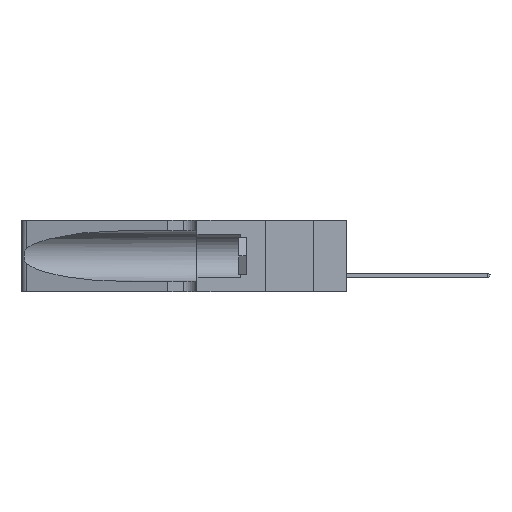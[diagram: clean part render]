
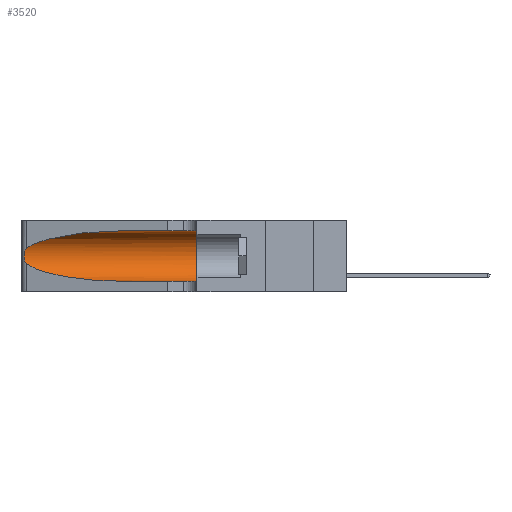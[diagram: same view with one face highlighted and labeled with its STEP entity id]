
A CAD part, left-side view. The second image highlights one B-rep face of the part: STEP entity #3520.
In plain terms, the highlighted cylindrical face has radius 3.308 mm (diameter 6.617 mm), a partial arc.
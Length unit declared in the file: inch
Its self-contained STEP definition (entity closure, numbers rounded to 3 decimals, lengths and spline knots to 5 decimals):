
#1212 = VECTOR ( 'NONE', #15139, 39.37008 ) ;
#1886 =( BOUNDED_CURVE ( )  B_SPLINE_CURVE ( 3, ( #22516, #39188, #35856, #42507 ),
 .UNSPECIFIED., .F., .T. ) 
 B_SPLINE_CURVE_WITH_KNOTS ( ( 4, 4 ),
 ( 1.5708, 2.84003 ),
 .UNSPECIFIED. ) 
 CURVE ( )  GEOMETRIC_REPRESENTATION_ITEM ( )  RATIONAL_B_SPLINE_CURVE ( ( 1., 0.87, 0.87, 1. ) ) 
 REPRESENTATION_ITEM ( '' )  );
#2965 = FACE_OUTER_BOUND ( 'NONE', #38478, .T. ) ;
#3320 = ORIENTED_EDGE ( 'NONE', *, *, #29223, .T. ) ;
#3520 = ADVANCED_FACE ( 'NONE', ( #2965 ), #28859, .F. ) ;
#4287 = CARTESIAN_POINT ( 'NONE',  ( 0.18966, 0.96281, 0.05475 ) ) ;
#4423 = CARTESIAN_POINT ( 'NONE',  ( 0.1305, 0.35, 0.05475 ) ) ;
#4901 = CARTESIAN_POINT ( 'NONE',  ( 0.26017, 1.23833, 0.17102 ) ) ;
#5806 = VERTEX_POINT ( 'NONE', #4423 ) ;
#6596 = DIRECTION ( 'NONE',  ( 0., 1., 0. ) ) ;
#6726 = CARTESIAN_POINT ( 'NONE',  ( 0.1305, 0.35, 0.185 ) ) ;
#7223 = CARTESIAN_POINT ( 'NONE',  ( 0.1305, 1.61858, 0.31525 ) ) ;
#7584 = EDGE_CURVE ( 'NONE', #34844, #7941, #1886, .T. ) ;
#7763 =( BOUNDED_CURVE ( )  B_SPLINE_CURVE ( 3, ( #33825, #10805, #4287, #20912 ),
 .UNSPECIFIED., .F., .F. ) 
 B_SPLINE_CURVE_WITH_KNOTS ( ( 4, 4 ),
 ( 3.44316, 4.71239 ),
 .UNSPECIFIED. ) 
 CURVE ( )  GEOMETRIC_REPRESENTATION_ITEM ( )  RATIONAL_B_SPLINE_CURVE ( ( 1., 0.87, 0.87, 1. ) ) 
 REPRESENTATION_ITEM ( '' )  );
#7941 = VERTEX_POINT ( 'NONE', #16054 ) ;
#8264 = CARTESIAN_POINT ( 'NONE',  ( 0.25639, 1.23186, 0.15144 ) ) ;
#8314 = CARTESIAN_POINT ( 'NONE',  ( 0.1305, 0.35, 0.31525 ) ) ;
#9198 = VERTEX_POINT ( 'NONE', #40824 ) ;
#10805 = CARTESIAN_POINT ( 'NONE',  ( 0.2373, 1.15595, 0.08982 ) ) ;
#10886 = VECTOR ( 'NONE', #20127, 39.37008 ) ;
#11933 = AXIS2_PLACEMENT_3D ( 'NONE', #38541, #35711, #20340 ) ;
#12037 = CARTESIAN_POINT ( 'NONE',  ( 0.26075, 1.23896, 0.19203 ) ) ;
#15139 = DIRECTION ( 'NONE',  ( 0., -1., 0. ) ) ;
#15474 = CARTESIAN_POINT ( 'NONE',  ( 0.25639, 1.23184, 0.21858 ) ) ;
#15624 = ORIENTED_EDGE ( 'NONE', *, *, #26979, .T. ) ;
#15671 = VERTEX_POINT ( 'NONE', #30046 ) ;
#16045 = ORIENTED_EDGE ( 'NONE', *, *, #30670, .T. ) ;
#16054 = CARTESIAN_POINT ( 'NONE',  ( 0.25487, 1.22718, 0.22369 ) ) ;
#16184 = ORIENTED_EDGE ( 'NONE', *, *, #7584, .T. ) ;
#16254 = EDGE_CURVE ( 'NONE', #34844, #33401, #18668, .T. ) ;
#17661 = CARTESIAN_POINT ( 'NONE',  ( 0.1305, 0.72297, 0.31525 ) ) ;
#18661 = CARTESIAN_POINT ( 'NONE',  ( 0.25555, 1.22993, 0.14849 ) ) ;
#18668 = LINE ( 'NONE', #7223, #10886 ) ;
#18811 = EDGE_CURVE ( 'NONE', #33401, #5806, #36048, .T. ) ;
#18915 = LINE ( 'NONE', #35158, #1212 ) ;
#20127 = DIRECTION ( 'NONE',  ( 0., -1., 0. ) ) ;
#20340 = DIRECTION ( 'NONE',  ( 0., 0., -1. ) ) ;
#20912 = CARTESIAN_POINT ( 'NONE',  ( 0.1305, 0.72297, 0.05475 ) ) ;
#21403 = CARTESIAN_POINT ( 'NONE',  ( 0.25789, 1.23486, 0.15765 ) ) ;
#21866 = CARTESIAN_POINT ( 'NONE',  ( 0.25854, 1.2359, 0.20912 ) ) ;
#22516 = CARTESIAN_POINT ( 'NONE',  ( 0.1305, 0.72297, 0.31525 ) ) ;
#25321 = CARTESIAN_POINT ( 'NONE',  ( 0.26018, 1.23835, 0.19895 ) ) ;
#25450 = AXIS2_PLACEMENT_3D ( 'NONE', #6726, #6596, #32948 ) ;
#26979 = EDGE_CURVE ( 'NONE', #15671, #9198, #7763, .T. ) ;
#28859 = CYLINDRICAL_SURFACE ( 'NONE', #11933, 0.13025 ) ;
#29223 = EDGE_CURVE ( 'NONE', #7941, #15671, #29593, .T. ) ;
#29593 = B_SPLINE_CURVE_WITH_KNOTS ( 'NONE', 3,
 ( #31578, #35346, #15474, #41717, #21866, #25321, #12037, #41264, #4901, #41417, #21403, #8264, #18661, #41856 ),
 .UNSPECIFIED., .F., .F.,
 ( 4, 2, 2, 2, 2, 2, 4 ),
 ( 0., 0.00027, 0.00053, 0.00107, 0.0016, 0.00187, 0.00214 ),
 .UNSPECIFIED. ) ;
#30046 = CARTESIAN_POINT ( 'NONE',  ( 0.25487, 1.22718, 0.14631 ) ) ;
#30174 = ORIENTED_EDGE ( 'NONE', *, *, #18811, .F. ) ;
#30670 = EDGE_CURVE ( 'NONE', #9198, #5806, #18915, .T. ) ;
#31578 = CARTESIAN_POINT ( 'NONE',  ( 0.25487, 1.22718, 0.22369 ) ) ;
#32948 = DIRECTION ( 'NONE',  ( 0., 0., 1. ) ) ;
#33401 = VERTEX_POINT ( 'NONE', #8314 ) ;
#33825 = CARTESIAN_POINT ( 'NONE',  ( 0.25487, 1.22718, 0.14631 ) ) ;
#34844 = VERTEX_POINT ( 'NONE', #17661 ) ;
#35158 = CARTESIAN_POINT ( 'NONE',  ( 0.1305, 1.61858, 0.05475 ) ) ;
#35346 = CARTESIAN_POINT ( 'NONE',  ( 0.25555, 1.22994, 0.2215 ) ) ;
#35711 = DIRECTION ( 'NONE',  ( 0., -1., 0. ) ) ;
#35856 = CARTESIAN_POINT ( 'NONE',  ( 0.2373, 1.15595, 0.28018 ) ) ;
#36048 = CIRCLE ( 'NONE', #25450, 0.13025 ) ;
#38478 = EDGE_LOOP ( 'NONE', ( #16184, #3320, #15624, #16045, #30174, #42156 ) ) ;
#38541 = CARTESIAN_POINT ( 'NONE',  ( 0.1305, 1.61858, 0.185 ) ) ;
#39188 = CARTESIAN_POINT ( 'NONE',  ( 0.18966, 0.96281, 0.31525 ) ) ;
#40824 = CARTESIAN_POINT ( 'NONE',  ( 0.1305, 0.72297, 0.05475 ) ) ;
#41264 = CARTESIAN_POINT ( 'NONE',  ( 0.26075, 1.23896, 0.178 ) ) ;
#41417 = CARTESIAN_POINT ( 'NONE',  ( 0.25856, 1.23593, 0.16098 ) ) ;
#41717 = CARTESIAN_POINT ( 'NONE',  ( 0.25787, 1.23484, 0.2124 ) ) ;
#41856 = CARTESIAN_POINT ( 'NONE',  ( 0.25487, 1.22718, 0.14631 ) ) ;
#42156 = ORIENTED_EDGE ( 'NONE', *, *, #16254, .F. ) ;
#42507 = CARTESIAN_POINT ( 'NONE',  ( 0.25487, 1.22718, 0.22369 ) ) ;
